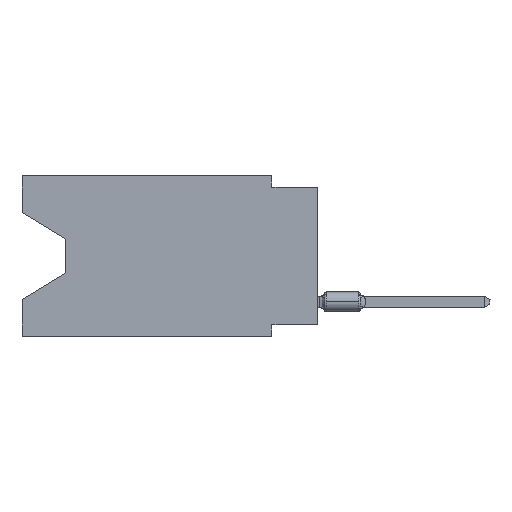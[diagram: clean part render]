
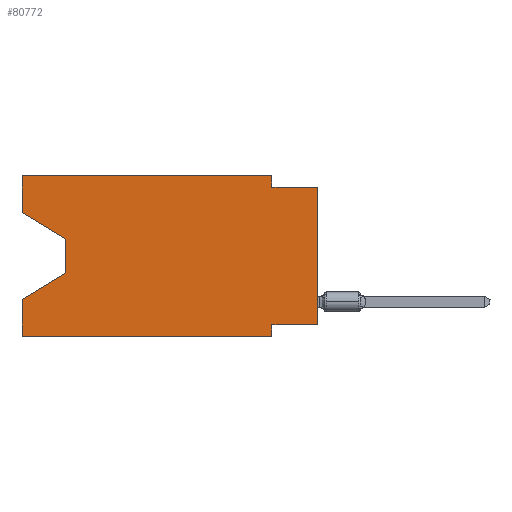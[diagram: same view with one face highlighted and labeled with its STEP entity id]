
A CAD part, left-side view. The second image highlights one B-rep face of the part: STEP entity #80772.
In plain terms, the highlighted planar face has unit normal (-1, 0, 0).
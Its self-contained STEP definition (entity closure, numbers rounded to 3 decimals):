
#689 = DIRECTION ( 'NONE',  ( 0., 0., 1. ) ) ;
#764 = ORIENTED_EDGE ( 'NONE', *, *, #90627, .F. ) ;
#886 = EDGE_CURVE ( 'NONE', #26515, #36476, #105679, .T. ) ;
#1452 = CARTESIAN_POINT ( 'NONE',  ( 0., 16.383, -2.038 ) ) ;
#4492 = DIRECTION ( 'NONE',  ( 0., 0., -1. ) ) ;
#5288 = VECTOR ( 'NONE', #49622, 1000. ) ;
#5496 = EDGE_CURVE ( 'NONE', #20959, #90509, #69067, .T. ) ;
#5557 = VECTOR ( 'NONE', #82100, 1000. ) ;
#7348 = ORIENTED_EDGE ( 'NONE', *, *, #31404, .T. ) ;
#7441 = CARTESIAN_POINT ( 'NONE',  ( 0., 13.97, -5.385 ) ) ;
#8293 = LINE ( 'NONE', #40707, #5288 ) ;
#8405 = VECTOR ( 'NONE', #36926, 1000. ) ;
#8638 = VERTEX_POINT ( 'NONE', #65904 ) ;
#8656 = CARTESIAN_POINT ( 'NONE',  ( 0., 13.97, -5.385 ) ) ;
#10339 = EDGE_CURVE ( 'NONE', #16231, #50725, #14453, .T. ) ;
#11949 = LINE ( 'NONE', #47105, #85312 ) ;
#13618 = PLANE ( 'NONE',  #70282 ) ;
#14453 = LINE ( 'NONE', #57398, #17993 ) ;
#15926 = LINE ( 'NONE', #50518, #48664 ) ;
#16231 = VERTEX_POINT ( 'NONE', #54085 ) ;
#17641 = VECTOR ( 'NONE', #689, 1000. ) ;
#17993 = VECTOR ( 'NONE', #75231, 1000. ) ;
#20959 = VERTEX_POINT ( 'NONE', #39550 ) ;
#21197 = CARTESIAN_POINT ( 'NONE',  ( 0., 2.54, -8.89 ) ) ;
#23171 = ORIENTED_EDGE ( 'NONE', *, *, #24262, .T. ) ;
#23247 = CARTESIAN_POINT ( 'NONE',  ( 0., 16.383, -2.038 ) ) ;
#23626 = LINE ( 'NONE', #7441, #42711 ) ;
#24262 = EDGE_CURVE ( 'NONE', #29552, #50725, #15926, .T. ) ;
#24704 = DIRECTION ( 'NONE',  ( 0., 0.855, -0.519 ) ) ;
#26317 = VERTEX_POINT ( 'NONE', #36135 ) ;
#26515 = VERTEX_POINT ( 'NONE', #23247 ) ;
#29552 = VERTEX_POINT ( 'NONE', #98678 ) ;
#31110 = ORIENTED_EDGE ( 'NONE', *, *, #886, .T. ) ;
#31404 = EDGE_CURVE ( 'NONE', #20959, #90676, #8293, .T. ) ;
#32407 = ORIENTED_EDGE ( 'NONE', *, *, #108322, .F. ) ;
#33168 = ORIENTED_EDGE ( 'NONE', *, *, #5496, .F. ) ;
#33417 = DIRECTION ( 'NONE',  ( 0., 0., 1. ) ) ;
#33500 = VERTEX_POINT ( 'NONE', #61651 ) ;
#34646 = ORIENTED_EDGE ( 'NONE', *, *, #108640, .T. ) ;
#36135 = CARTESIAN_POINT ( 'NONE',  ( 0., 2.54, 0. ) ) ;
#36476 = VERTEX_POINT ( 'NONE', #42818 ) ;
#36926 = DIRECTION ( 'NONE',  ( 0., -1., 0. ) ) ;
#39074 = ORIENTED_EDGE ( 'NONE', *, *, #101962, .T. ) ;
#39550 = CARTESIAN_POINT ( 'NONE',  ( 0., 16.383, -8.89 ) ) ;
#39853 = FACE_OUTER_BOUND ( 'NONE', #98353, .T. ) ;
#40707 = CARTESIAN_POINT ( 'NONE',  ( 0., 16.383, -8.89 ) ) ;
#40990 = EDGE_CURVE ( 'NONE', #29552, #33500, #11949, .T. ) ;
#42711 = VECTOR ( 'NONE', #24704, 1000. ) ;
#42818 = CARTESIAN_POINT ( 'NONE',  ( 0., 13.97, -3.505 ) ) ;
#43075 = LINE ( 'NONE', #77074, #17641 ) ;
#46093 = VERTEX_POINT ( 'NONE', #8656 ) ;
#47105 = CARTESIAN_POINT ( 'NONE',  ( 0., 0., -8.255 ) ) ;
#48664 = VECTOR ( 'NONE', #49976, 1000. ) ;
#49622 = DIRECTION ( 'NONE',  ( 0., -1., 0. ) ) ;
#49976 = DIRECTION ( 'NONE',  ( 0., 0., 1. ) ) ;
#50518 = CARTESIAN_POINT ( 'NONE',  ( 0., 0., 0. ) ) ;
#50725 = VERTEX_POINT ( 'NONE', #90931 ) ;
#52895 = ORIENTED_EDGE ( 'NONE', *, *, #10339, .F. ) ;
#54085 = CARTESIAN_POINT ( 'NONE',  ( 0., 2.54, -0.635 ) ) ;
#55342 = CARTESIAN_POINT ( 'NONE',  ( 0., 16.383, -6.852 ) ) ;
#55887 = LINE ( 'NONE', #98280, #5557 ) ;
#56014 = CARTESIAN_POINT ( 'NONE',  ( 0., 16.383, 0. ) ) ;
#57398 = CARTESIAN_POINT ( 'NONE',  ( 0., 0., -0.635 ) ) ;
#59183 = ORIENTED_EDGE ( 'NONE', *, *, #86751, .F. ) ;
#61651 = CARTESIAN_POINT ( 'NONE',  ( 0., 2.54, -8.255 ) ) ;
#62991 = VECTOR ( 'NONE', #4492, 1000. ) ;
#64393 = DIRECTION ( 'NONE',  ( 1., 0., 0. ) ) ;
#65904 = CARTESIAN_POINT ( 'NONE',  ( 0., 16.383, 0. ) ) ;
#66906 = LINE ( 'NONE', #84169, #96901 ) ;
#68526 = CARTESIAN_POINT ( 'NONE',  ( 0., 16.383, 0. ) ) ;
#69067 = LINE ( 'NONE', #68526, #81311 ) ;
#70282 = AXIS2_PLACEMENT_3D ( 'NONE', #56014, #64393, #100050 ) ;
#73088 = ORIENTED_EDGE ( 'NONE', *, *, #40990, .F. ) ;
#74838 = CARTESIAN_POINT ( 'NONE',  ( 0., 2.54, -8.89 ) ) ;
#75231 = DIRECTION ( 'NONE',  ( 0., -1., 0. ) ) ;
#77074 = CARTESIAN_POINT ( 'NONE',  ( 0., 16.383, 0. ) ) ;
#79303 = CARTESIAN_POINT ( 'NONE',  ( 0., 16.383, 0. ) ) ;
#80772 = ADVANCED_FACE ( 'NONE', ( #39853 ), #13618, .F. ) ;
#81311 = VECTOR ( 'NONE', #33417, 1000. ) ;
#82100 = DIRECTION ( 'NONE',  ( 0., 0., -1. ) ) ;
#84169 = CARTESIAN_POINT ( 'NONE',  ( 0., 13.97, -3.505 ) ) ;
#85312 = VECTOR ( 'NONE', #87264, 1000. ) ;
#86751 = EDGE_CURVE ( 'NONE', #26515, #8638, #43075, .T. ) ;
#87264 = DIRECTION ( 'NONE',  ( 0., 1., 0. ) ) ;
#89855 = LINE ( 'NONE', #79303, #8405 ) ;
#90509 = VERTEX_POINT ( 'NONE', #55342 ) ;
#90627 = EDGE_CURVE ( 'NONE', #26317, #16231, #55887, .T. ) ;
#90676 = VERTEX_POINT ( 'NONE', #74838 ) ;
#90931 = CARTESIAN_POINT ( 'NONE',  ( 0., 0., -0.635 ) ) ;
#96134 = EDGE_CURVE ( 'NONE', #8638, #26317, #89855, .T. ) ;
#96901 = VECTOR ( 'NONE', #103083, 1000. ) ;
#97328 = DIRECTION ( 'NONE',  ( 0., -0.855, -0.519 ) ) ;
#97611 = LINE ( 'NONE', #21197, #62991 ) ;
#98280 = CARTESIAN_POINT ( 'NONE',  ( 0., 2.54, 0. ) ) ;
#98353 = EDGE_LOOP ( 'NONE', ( #31110, #34646, #39074, #33168, #7348, #32407, #73088, #23171, #52895, #764, #108190, #59183 ) ) ;
#98614 = VECTOR ( 'NONE', #97328, 1000. ) ;
#98678 = CARTESIAN_POINT ( 'NONE',  ( 0., 0., -8.255 ) ) ;
#100050 = DIRECTION ( 'NONE',  ( 0., 0., -1. ) ) ;
#101962 = EDGE_CURVE ( 'NONE', #46093, #90509, #23626, .T. ) ;
#103083 = DIRECTION ( 'NONE',  ( 0., 0., -1. ) ) ;
#105679 = LINE ( 'NONE', #1452, #98614 ) ;
#108190 = ORIENTED_EDGE ( 'NONE', *, *, #96134, .F. ) ;
#108322 = EDGE_CURVE ( 'NONE', #33500, #90676, #97611, .T. ) ;
#108640 = EDGE_CURVE ( 'NONE', #36476, #46093, #66906, .T. ) ;
